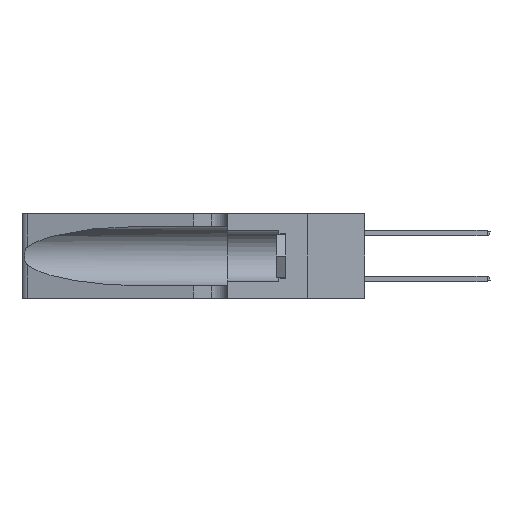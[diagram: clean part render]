
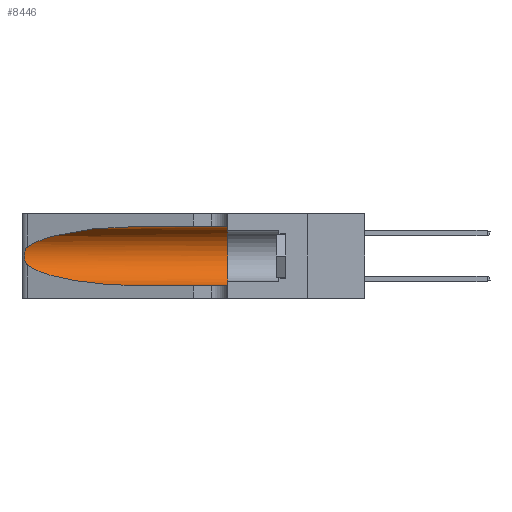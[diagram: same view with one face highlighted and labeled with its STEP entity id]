
A CAD part, left-side view. The second image highlights one B-rep face of the part: STEP entity #8446.
In plain terms, the highlighted cylindrical face has radius 3.308 mm (diameter 6.617 mm), a partial arc.
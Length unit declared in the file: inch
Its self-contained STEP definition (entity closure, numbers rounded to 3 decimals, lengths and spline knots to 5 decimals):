
#133 = AXIS2_PLACEMENT_3D ( 'NONE', #2174, #4792, #21336 ) ;
#238 = CIRCLE ( 'NONE', #16691, 0.13025 ) ;
#500 = VERTEX_POINT ( 'NONE', #1711 ) ;
#521 = B_SPLINE_CURVE_WITH_KNOTS ( 'NONE', 3,
 ( #30656, #24368, #10824, #23268, #10087, #28602, #12827, #9604, #12353, #34037, #28836, #15320, #4245, #6981 ),
 .UNSPECIFIED., .F., .F.,
 ( 4, 2, 2, 2, 2, 2, 4 ),
 ( 0., 0.00027, 0.00053, 0.00107, 0.0016, 0.00187, 0.00214 ),
 .UNSPECIFIED. ) ;
#970 =( BOUNDED_CURVE ( )  B_SPLINE_CURVE ( 3, ( #21428, #2386, #7975, #7627 ),
 .UNSPECIFIED., .F., .T. ) 
 B_SPLINE_CURVE_WITH_KNOTS ( ( 4, 4 ),
 ( 3.44316, 4.71239 ),
 .UNSPECIFIED. ) 
 CURVE ( )  GEOMETRIC_REPRESENTATION_ITEM ( )  RATIONAL_B_SPLINE_CURVE ( ( 1., 0.87, 0.87, 1. ) ) 
 REPRESENTATION_ITEM ( '' )  );
#1031 = ORIENTED_EDGE ( 'NONE', *, *, #3028, .T. ) ;
#1711 = CARTESIAN_POINT ( 'NONE',  ( 0.25487, 1.22718, 0.14631 ) ) ;
#1849 = CARTESIAN_POINT ( 'NONE',  ( 0.1305, 0.35, 0.05475 ) ) ;
#2174 = CARTESIAN_POINT ( 'NONE',  ( 0.1305, 1.61858, 0.185 ) ) ;
#2386 = CARTESIAN_POINT ( 'NONE',  ( 0.2373, 1.15595, 0.08982 ) ) ;
#2727 = EDGE_CURVE ( 'NONE', #27255, #500, #521, .T. ) ;
#3011 = VECTOR ( 'NONE', #33124, 39.37008 ) ;
#3028 = EDGE_CURVE ( 'NONE', #28827, #27255, #6832, .T. ) ;
#4245 = CARTESIAN_POINT ( 'NONE',  ( 0.25555, 1.22993, 0.14849 ) ) ;
#4592 = EDGE_LOOP ( 'NONE', ( #1031, #22638, #29058, #25357, #25758, #12135 ) ) ;
#4699 = VERTEX_POINT ( 'NONE', #1849 ) ;
#4792 = DIRECTION ( 'NONE',  ( 0., -1., 0. ) ) ;
#6303 = CARTESIAN_POINT ( 'NONE',  ( 0.2373, 1.15595, 0.28018 ) ) ;
#6438 = DIRECTION ( 'NONE',  ( 0., -1., 0. ) ) ;
#6832 =( BOUNDED_CURVE ( )  B_SPLINE_CURVE ( 3, ( #33744, #17543, #6303, #34068 ),
 .UNSPECIFIED., .F., .F. ) 
 B_SPLINE_CURVE_WITH_KNOTS ( ( 4, 4 ),
 ( 1.5708, 2.84003 ),
 .UNSPECIFIED. ) 
 CURVE ( )  GEOMETRIC_REPRESENTATION_ITEM ( )  RATIONAL_B_SPLINE_CURVE ( ( 1., 0.87, 0.87, 1. ) ) 
 REPRESENTATION_ITEM ( '' )  );
#6981 = CARTESIAN_POINT ( 'NONE',  ( 0.25487, 1.22718, 0.14631 ) ) ;
#7393 = CARTESIAN_POINT ( 'NONE',  ( 0.1305, 0.72297, 0.05475 ) ) ;
#7627 = CARTESIAN_POINT ( 'NONE',  ( 0.1305, 0.72297, 0.05475 ) ) ;
#7975 = CARTESIAN_POINT ( 'NONE',  ( 0.18966, 0.96281, 0.05475 ) ) ;
#8302 = VERTEX_POINT ( 'NONE', #9552 ) ;
#8446 = ADVANCED_FACE ( 'NONE', ( #20335 ), #24584, .F. ) ;
#9552 = CARTESIAN_POINT ( 'NONE',  ( 0.1305, 0.35, 0.31525 ) ) ;
#9604 = CARTESIAN_POINT ( 'NONE',  ( 0.26075, 1.23896, 0.178 ) ) ;
#9976 = VECTOR ( 'NONE', #6438, 39.37008 ) ;
#10087 = CARTESIAN_POINT ( 'NONE',  ( 0.25854, 1.2359, 0.20912 ) ) ;
#10824 = CARTESIAN_POINT ( 'NONE',  ( 0.25639, 1.23184, 0.21858 ) ) ;
#11092 = EDGE_CURVE ( 'NONE', #500, #14701, #970, .T. ) ;
#11536 = DIRECTION ( 'NONE',  ( 0., 1., 0. ) ) ;
#12135 = ORIENTED_EDGE ( 'NONE', *, *, #18269, .F. ) ;
#12353 = CARTESIAN_POINT ( 'NONE',  ( 0.26017, 1.23833, 0.17102 ) ) ;
#12827 = CARTESIAN_POINT ( 'NONE',  ( 0.26075, 1.23896, 0.19203 ) ) ;
#13677 = LINE ( 'NONE', #18100, #3011 ) ;
#14701 = VERTEX_POINT ( 'NONE', #7393 ) ;
#14846 = EDGE_CURVE ( 'NONE', #14701, #4699, #20598, .T. ) ;
#15320 = CARTESIAN_POINT ( 'NONE',  ( 0.25639, 1.23186, 0.15144 ) ) ;
#16691 = AXIS2_PLACEMENT_3D ( 'NONE', #22559, #11536, #30643 ) ;
#17543 = CARTESIAN_POINT ( 'NONE',  ( 0.18966, 0.96281, 0.31525 ) ) ;
#17647 = CARTESIAN_POINT ( 'NONE',  ( 0.1305, 1.61858, 0.05475 ) ) ;
#18100 = CARTESIAN_POINT ( 'NONE',  ( 0.1305, 1.61858, 0.31525 ) ) ;
#18269 = EDGE_CURVE ( 'NONE', #28827, #8302, #13677, .T. ) ;
#20335 = FACE_OUTER_BOUND ( 'NONE', #4592, .T. ) ;
#20598 = LINE ( 'NONE', #17647, #9976 ) ;
#21336 = DIRECTION ( 'NONE',  ( 0., 0., -1. ) ) ;
#21428 = CARTESIAN_POINT ( 'NONE',  ( 0.25487, 1.22718, 0.14631 ) ) ;
#22559 = CARTESIAN_POINT ( 'NONE',  ( 0.1305, 0.35, 0.185 ) ) ;
#22638 = ORIENTED_EDGE ( 'NONE', *, *, #2727, .T. ) ;
#23268 = CARTESIAN_POINT ( 'NONE',  ( 0.25787, 1.23484, 0.2124 ) ) ;
#24368 = CARTESIAN_POINT ( 'NONE',  ( 0.25555, 1.22994, 0.2215 ) ) ;
#24584 = CYLINDRICAL_SURFACE ( 'NONE', #133, 0.13025 ) ;
#25357 = ORIENTED_EDGE ( 'NONE', *, *, #14846, .T. ) ;
#25758 = ORIENTED_EDGE ( 'NONE', *, *, #30157, .F. ) ;
#27255 = VERTEX_POINT ( 'NONE', #27740 ) ;
#27740 = CARTESIAN_POINT ( 'NONE',  ( 0.25487, 1.22718, 0.22369 ) ) ;
#28602 = CARTESIAN_POINT ( 'NONE',  ( 0.26018, 1.23835, 0.19895 ) ) ;
#28827 = VERTEX_POINT ( 'NONE', #33017 ) ;
#28836 = CARTESIAN_POINT ( 'NONE',  ( 0.25789, 1.23486, 0.15765 ) ) ;
#29058 = ORIENTED_EDGE ( 'NONE', *, *, #11092, .T. ) ;
#30157 = EDGE_CURVE ( 'NONE', #8302, #4699, #238, .T. ) ;
#30643 = DIRECTION ( 'NONE',  ( 0., 0., 1. ) ) ;
#30656 = CARTESIAN_POINT ( 'NONE',  ( 0.25487, 1.22718, 0.22369 ) ) ;
#33017 = CARTESIAN_POINT ( 'NONE',  ( 0.1305, 0.72297, 0.31525 ) ) ;
#33124 = DIRECTION ( 'NONE',  ( 0., -1., 0. ) ) ;
#33744 = CARTESIAN_POINT ( 'NONE',  ( 0.1305, 0.72297, 0.31525 ) ) ;
#34037 = CARTESIAN_POINT ( 'NONE',  ( 0.25856, 1.23593, 0.16098 ) ) ;
#34068 = CARTESIAN_POINT ( 'NONE',  ( 0.25487, 1.22718, 0.22369 ) ) ;
